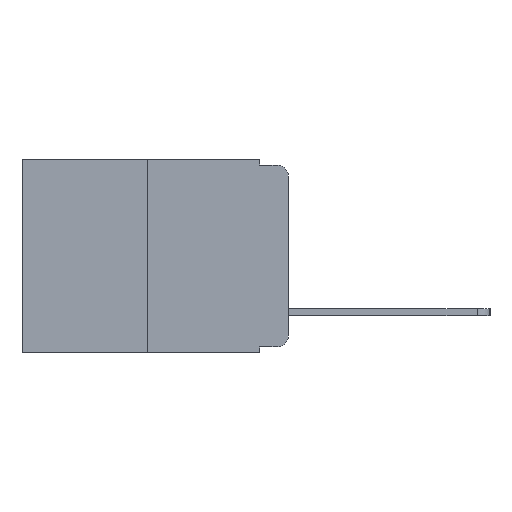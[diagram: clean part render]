
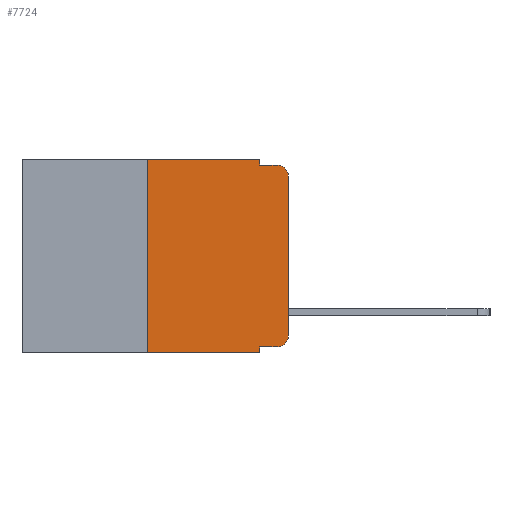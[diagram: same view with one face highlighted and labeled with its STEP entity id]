
A CAD part, left-side view. The second image highlights one B-rep face of the part: STEP entity #7724.
In plain terms, the highlighted planar face has unit normal (-1, 0, 0).
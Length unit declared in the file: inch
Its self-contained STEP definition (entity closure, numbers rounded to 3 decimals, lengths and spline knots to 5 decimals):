
#48 = DIRECTION ( 'NONE',  ( 1., 0., 0. ) ) ;
#188 = DIRECTION ( 'NONE',  ( 0., -1., 0. ) ) ;
#210 = AXIS2_PLACEMENT_3D ( 'NONE', #3407, #10034, #4419 ) ;
#277 = CARTESIAN_POINT ( 'NONE',  ( 0., 0.02, -0.313 ) ) ;
#423 = LINE ( 'NONE', #7965, #10496 ) ;
#972 = VERTEX_POINT ( 'NONE', #3935 ) ;
#981 = LINE ( 'NONE', #6022, #8250 ) ;
#1086 = ORIENTED_EDGE ( 'NONE', *, *, #11267, .F. ) ;
#1349 = DIRECTION ( 'NONE',  ( 0., 0., -1. ) ) ;
#1430 = LINE ( 'NONE', #8784, #11059 ) ;
#1588 = ORIENTED_EDGE ( 'NONE', *, *, #7857, .T. ) ;
#1646 = VERTEX_POINT ( 'NONE', #6464 ) ;
#1945 = ORIENTED_EDGE ( 'NONE', *, *, #7805, .F. ) ;
#2022 = CARTESIAN_POINT ( 'NONE',  ( 0., 0.051, -0.01 ) ) ;
#2663 = LINE ( 'NONE', #5717, #8110 ) ;
#2755 = ORIENTED_EDGE ( 'NONE', *, *, #6339, .F. ) ;
#3056 = AXIS2_PLACEMENT_3D ( 'NONE', #277, #7303, #1349 ) ;
#3407 = CARTESIAN_POINT ( 'NONE',  ( 0., 0.02, -0.03 ) ) ;
#3411 = VECTOR ( 'NONE', #188, 39.37008 ) ;
#3846 = DIRECTION ( 'NONE',  ( 0., 0., -1. ) ) ;
#3935 = CARTESIAN_POINT ( 'NONE',  ( 0., 0.051, 0. ) ) ;
#4419 = DIRECTION ( 'NONE',  ( 0., 0., -1. ) ) ;
#4477 = ORIENTED_EDGE ( 'NONE', *, *, #5742, .F. ) ;
#4516 = VERTEX_POINT ( 'NONE', #2022 ) ;
#4724 = DIRECTION ( 'NONE',  ( 0., -1., 0. ) ) ;
#4858 = CARTESIAN_POINT ( 'NONE',  ( 0., 0.051, 0. ) ) ;
#4864 = CARTESIAN_POINT ( 'NONE',  ( 0., 0.051, -0.343 ) ) ;
#5178 = DIRECTION ( 'NONE',  ( 0., 0., 1. ) ) ;
#5463 = ORIENTED_EDGE ( 'NONE', *, *, #7873, .T. ) ;
#5509 = CARTESIAN_POINT ( 'NONE',  ( 0., 0.02, -0.01 ) ) ;
#5510 = CARTESIAN_POINT ( 'NONE',  ( 0., 0.051, -0.333 ) ) ;
#5543 = EDGE_CURVE ( 'NONE', #8054, #11949, #2663, .T. ) ;
#5692 = CARTESIAN_POINT ( 'NONE',  ( 0., 0.051, -0.333 ) ) ;
#5717 = CARTESIAN_POINT ( 'NONE',  ( 0., 0.473, -0.343 ) ) ;
#5735 = CIRCLE ( 'NONE', #3056, 0.02 ) ;
#5742 = EDGE_CURVE ( 'NONE', #972, #4516, #981, .T. ) ;
#6022 = CARTESIAN_POINT ( 'NONE',  ( 0., 0.051, 0. ) ) ;
#6051 = LINE ( 'NONE', #9035, #3411 ) ;
#6339 = EDGE_CURVE ( 'NONE', #6756, #11949, #9110, .T. ) ;
#6464 = CARTESIAN_POINT ( 'NONE',  ( 0., 0., -0.03 ) ) ;
#6756 = VERTEX_POINT ( 'NONE', #5510 ) ;
#6764 = ORIENTED_EDGE ( 'NONE', *, *, #5543, .T. ) ;
#6918 = CARTESIAN_POINT ( 'NONE',  ( 0., 0., -0.313 ) ) ;
#6961 = DIRECTION ( 'NONE',  ( 0., -1., 0. ) ) ;
#7113 = DIRECTION ( 'NONE',  ( 0., 0., -1. ) ) ;
#7303 = DIRECTION ( 'NONE',  ( -1., 0., 0. ) ) ;
#7434 = VERTEX_POINT ( 'NONE', #11211 ) ;
#7661 = VECTOR ( 'NONE', #3846, 39.37008 ) ;
#7724 = ADVANCED_FACE ( 'NONE', ( #11797 ), #8924, .F. ) ;
#7805 = EDGE_CURVE ( 'NONE', #10001, #972, #6051, .T. ) ;
#7857 = EDGE_CURVE ( 'NONE', #1646, #10273, #10364, .T. ) ;
#7873 = EDGE_CURVE ( 'NONE', #7434, #10560, #5735, .T. ) ;
#7890 = ORIENTED_EDGE ( 'NONE', *, *, #10651, .T. ) ;
#7897 = CARTESIAN_POINT ( 'NONE',  ( 0., 0.25, 0. ) ) ;
#7940 = EDGE_LOOP ( 'NONE', ( #7890, #1588, #8030, #4477, #1945, #1086, #6764, #2755, #8523, #5463 ) ) ;
#7965 = CARTESIAN_POINT ( 'NONE',  ( 0., 0., 0. ) ) ;
#8030 = ORIENTED_EDGE ( 'NONE', *, *, #10584, .F. ) ;
#8054 = VERTEX_POINT ( 'NONE', #12114 ) ;
#8073 = VECTOR ( 'NONE', #4724, 39.37008 ) ;
#8110 = VECTOR ( 'NONE', #12174, 39.37008 ) ;
#8250 = VECTOR ( 'NONE', #11533, 39.37008 ) ;
#8523 = ORIENTED_EDGE ( 'NONE', *, *, #9767, .T. ) ;
#8769 = VECTOR ( 'NONE', #12486, 39.37008 ) ;
#8784 = CARTESIAN_POINT ( 'NONE',  ( 0., 0.051, -0.01 ) ) ;
#8924 = PLANE ( 'NONE',  #12131 ) ;
#9035 = CARTESIAN_POINT ( 'NONE',  ( 0., 0.473, 0. ) ) ;
#9110 = LINE ( 'NONE', #4858, #7661 ) ;
#9767 = EDGE_CURVE ( 'NONE', #6756, #7434, #10788, .T. ) ;
#10001 = VERTEX_POINT ( 'NONE', #7897 ) ;
#10034 = DIRECTION ( 'NONE',  ( -1., 0., 0. ) ) ;
#10273 = VERTEX_POINT ( 'NONE', #5509 ) ;
#10364 = CIRCLE ( 'NONE', #210, 0.02 ) ;
#10496 = VECTOR ( 'NONE', #5178, 39.37008 ) ;
#10560 = VERTEX_POINT ( 'NONE', #6918 ) ;
#10584 = EDGE_CURVE ( 'NONE', #4516, #10273, #1430, .T. ) ;
#10651 = EDGE_CURVE ( 'NONE', #10560, #1646, #423, .T. ) ;
#10746 = CARTESIAN_POINT ( 'NONE',  ( 0., 0.473, 0. ) ) ;
#10788 = LINE ( 'NONE', #5692, #8073 ) ;
#11059 = VECTOR ( 'NONE', #6961, 39.37008 ) ;
#11194 = LINE ( 'NONE', #12527, #8769 ) ;
#11211 = CARTESIAN_POINT ( 'NONE',  ( 0., 0.02, -0.333 ) ) ;
#11267 = EDGE_CURVE ( 'NONE', #8054, #10001, #11194, .T. ) ;
#11533 = DIRECTION ( 'NONE',  ( 0., 0., -1. ) ) ;
#11797 = FACE_OUTER_BOUND ( 'NONE', #7940, .T. ) ;
#11949 = VERTEX_POINT ( 'NONE', #4864 ) ;
#12114 = CARTESIAN_POINT ( 'NONE',  ( 0., 0.25, -0.343 ) ) ;
#12131 = AXIS2_PLACEMENT_3D ( 'NONE', #10746, #48, #7113 ) ;
#12174 = DIRECTION ( 'NONE',  ( 0., -1., 0. ) ) ;
#12486 = DIRECTION ( 'NONE',  ( 0., 0., 1. ) ) ;
#12527 = CARTESIAN_POINT ( 'NONE',  ( 0., 0.25, 0. ) ) ;
